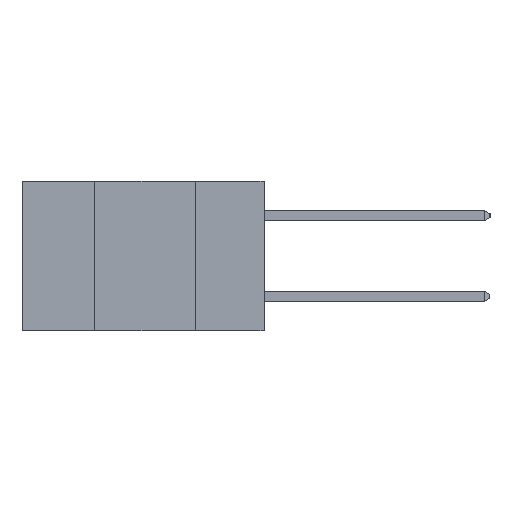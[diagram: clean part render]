
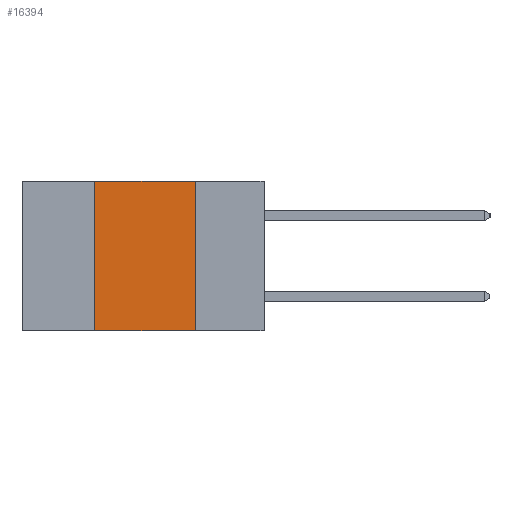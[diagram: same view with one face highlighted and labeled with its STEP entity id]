
A CAD part, left-side view. The second image highlights one B-rep face of the part: STEP entity #16394.
In plain terms, the highlighted planar face has unit normal (-1, 0, 0).
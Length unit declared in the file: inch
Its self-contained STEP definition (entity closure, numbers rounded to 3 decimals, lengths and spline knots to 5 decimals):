
#1253 = CARTESIAN_POINT ( 'NONE',  ( 0., 0.42, -0.37 ) ) ;
#1632 = LINE ( 'NONE', #1742, #22857 ) ;
#1730 = CARTESIAN_POINT ( 'NONE',  ( 0., 0.42, 0. ) ) ;
#1742 = CARTESIAN_POINT ( 'NONE',  ( 0., 0.6, -0.37 ) ) ;
#2392 = CARTESIAN_POINT ( 'NONE',  ( 0., 0.17, -0.37 ) ) ;
#4858 = CARTESIAN_POINT ( 'NONE',  ( 0., 0.6, 0. ) ) ;
#5583 = ORIENTED_EDGE ( 'NONE', *, *, #20383, .F. ) ;
#6684 = EDGE_CURVE ( 'NONE', #8251, #8148, #1632, .T. ) ;
#7176 = FACE_OUTER_BOUND ( 'NONE', #19005, .T. ) ;
#8127 = LINE ( 'NONE', #20733, #15659 ) ;
#8148 = VERTEX_POINT ( 'NONE', #11557 ) ;
#8251 = VERTEX_POINT ( 'NONE', #1253 ) ;
#11540 = DIRECTION ( 'NONE',  ( 0., -1., 0. ) ) ;
#11557 = CARTESIAN_POINT ( 'NONE',  ( 0., 0.17, -0.37 ) ) ;
#12249 = VERTEX_POINT ( 'NONE', #15666 ) ;
#12325 = VECTOR ( 'NONE', #11540, 39.37008 ) ;
#12425 = CARTESIAN_POINT ( 'NONE',  ( 0., 0.6, 0. ) ) ;
#12710 = DIRECTION ( 'NONE',  ( 0., 0., -1. ) ) ;
#13343 = ORIENTED_EDGE ( 'NONE', *, *, #6684, .T. ) ;
#13416 = LINE ( 'NONE', #4858, #12325 ) ;
#13742 = ORIENTED_EDGE ( 'NONE', *, *, #22373, .F. ) ;
#15033 = DIRECTION ( 'NONE',  ( 0., 0., 1. ) ) ;
#15659 = VECTOR ( 'NONE', #15033, 39.37008 ) ;
#15666 = CARTESIAN_POINT ( 'NONE',  ( 0., 0.17, 0. ) ) ;
#16394 = ADVANCED_FACE ( 'NONE', ( #7176 ), #19663, .F. ) ;
#17995 = DIRECTION ( 'NONE',  ( 0., -1., 0. ) ) ;
#18143 = DIRECTION ( 'NONE',  ( 0., 0., -1. ) ) ;
#18299 = LINE ( 'NONE', #2392, #18671 ) ;
#18671 = VECTOR ( 'NONE', #12710, 39.37008 ) ;
#19005 = EDGE_LOOP ( 'NONE', ( #5583, #21100, #13742, #13343 ) ) ;
#19289 = AXIS2_PLACEMENT_3D ( 'NONE', #12425, #21779, #18143 ) ;
#19663 = PLANE ( 'NONE',  #19289 ) ;
#19874 = VERTEX_POINT ( 'NONE', #1730 ) ;
#20129 = EDGE_CURVE ( 'NONE', #19874, #12249, #13416, .T. ) ;
#20383 = EDGE_CURVE ( 'NONE', #12249, #8148, #18299, .T. ) ;
#20733 = CARTESIAN_POINT ( 'NONE',  ( 0., 0.42, -0.37 ) ) ;
#21100 = ORIENTED_EDGE ( 'NONE', *, *, #20129, .F. ) ;
#21779 = DIRECTION ( 'NONE',  ( 1., 0., 0. ) ) ;
#22373 = EDGE_CURVE ( 'NONE', #8251, #19874, #8127, .T. ) ;
#22857 = VECTOR ( 'NONE', #17995, 39.37008 ) ;
